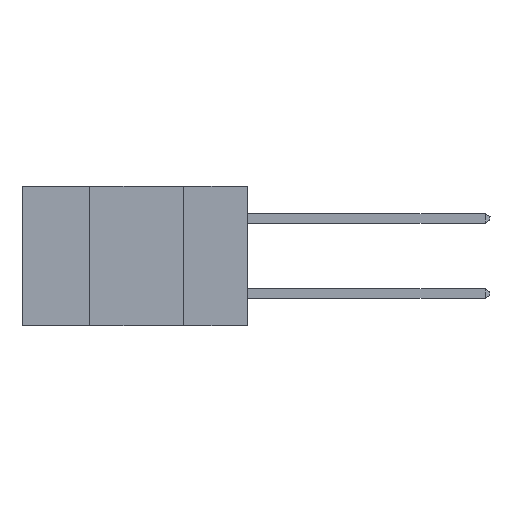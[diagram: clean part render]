
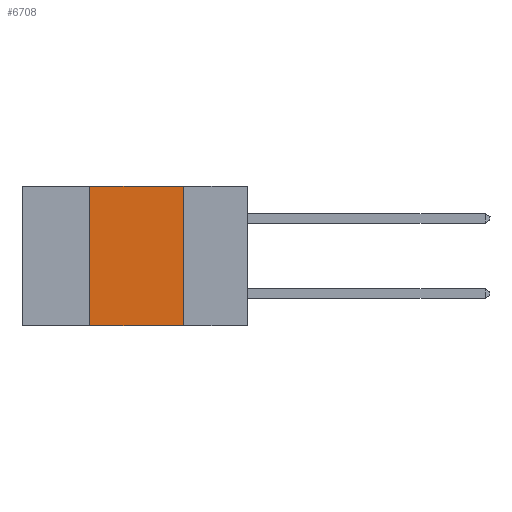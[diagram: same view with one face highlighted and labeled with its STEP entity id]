
A CAD part, left-side view. The second image highlights one B-rep face of the part: STEP entity #6708.
In plain terms, the highlighted planar face has unit normal (-1, 0, 0).
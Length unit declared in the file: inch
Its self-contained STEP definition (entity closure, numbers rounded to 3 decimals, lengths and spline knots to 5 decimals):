
#35 = VECTOR ( 'NONE', #3137, 39.37008 ) ;
#489 = VECTOR ( 'NONE', #10233, 39.37008 ) ;
#548 = DIRECTION ( 'NONE',  ( 0., 0., -1. ) ) ;
#591 = CARTESIAN_POINT ( 'NONE',  ( 0., 0.6, 0. ) ) ;
#878 = LINE ( 'NONE', #10620, #1305 ) ;
#1305 = VECTOR ( 'NONE', #11476, 39.37008 ) ;
#1320 = EDGE_LOOP ( 'NONE', ( #8663, #2267, #2986, #6158 ) ) ;
#2267 = ORIENTED_EDGE ( 'NONE', *, *, #6322, .F. ) ;
#2615 = LINE ( 'NONE', #5978, #35 ) ;
#2986 = ORIENTED_EDGE ( 'NONE', *, *, #9179, .F. ) ;
#3116 = VERTEX_POINT ( 'NONE', #8524 ) ;
#3121 = AXIS2_PLACEMENT_3D ( 'NONE', #591, #7042, #548 ) ;
#3137 = DIRECTION ( 'NONE',  ( 0., -1., 0. ) ) ;
#4412 = DIRECTION ( 'NONE',  ( 0., -1., 0. ) ) ;
#4889 = EDGE_CURVE ( 'NONE', #7775, #3116, #9311, .T. ) ;
#5065 = VECTOR ( 'NONE', #4412, 39.37008 ) ;
#5441 = CARTESIAN_POINT ( 'NONE',  ( 0., 0.17, 0. ) ) ;
#5978 = CARTESIAN_POINT ( 'NONE',  ( 0., 0.6, 0. ) ) ;
#6121 = PLANE ( 'NONE',  #3121 ) ;
#6136 = EDGE_CURVE ( 'NONE', #8139, #3116, #7382, .T. ) ;
#6158 = ORIENTED_EDGE ( 'NONE', *, *, #6136, .T. ) ;
#6322 = EDGE_CURVE ( 'NONE', #10238, #7775, #2615, .T. ) ;
#6519 = CARTESIAN_POINT ( 'NONE',  ( 0., 0.42, 0. ) ) ;
#6708 = ADVANCED_FACE ( 'NONE', ( #9098 ), #6121, .F. ) ;
#6889 = CARTESIAN_POINT ( 'NONE',  ( 0., 0.42, -0.37 ) ) ;
#7042 = DIRECTION ( 'NONE',  ( 1., 0., 0. ) ) ;
#7382 = LINE ( 'NONE', #8018, #5065 ) ;
#7775 = VERTEX_POINT ( 'NONE', #9919 ) ;
#8018 = CARTESIAN_POINT ( 'NONE',  ( 0., 0.6, -0.37 ) ) ;
#8139 = VERTEX_POINT ( 'NONE', #6889 ) ;
#8524 = CARTESIAN_POINT ( 'NONE',  ( 0., 0.17, -0.37 ) ) ;
#8663 = ORIENTED_EDGE ( 'NONE', *, *, #4889, .F. ) ;
#9098 = FACE_OUTER_BOUND ( 'NONE', #1320, .T. ) ;
#9179 = EDGE_CURVE ( 'NONE', #8139, #10238, #878, .T. ) ;
#9311 = LINE ( 'NONE', #5441, #489 ) ;
#9919 = CARTESIAN_POINT ( 'NONE',  ( 0., 0.17, 0. ) ) ;
#10233 = DIRECTION ( 'NONE',  ( 0., 0., -1. ) ) ;
#10238 = VERTEX_POINT ( 'NONE', #6519 ) ;
#10620 = CARTESIAN_POINT ( 'NONE',  ( 0., 0.42, 0. ) ) ;
#11476 = DIRECTION ( 'NONE',  ( 0., 0., 1. ) ) ;
